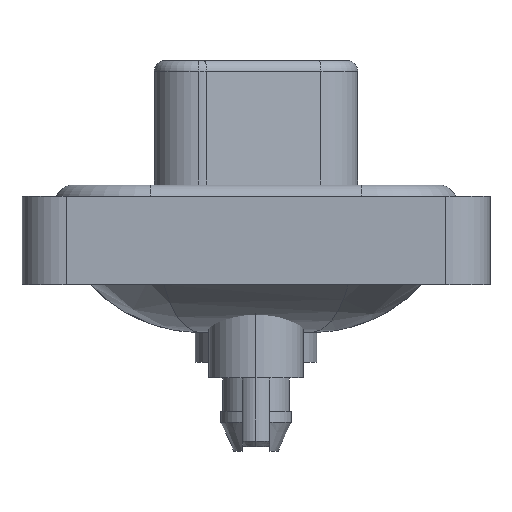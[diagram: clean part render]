
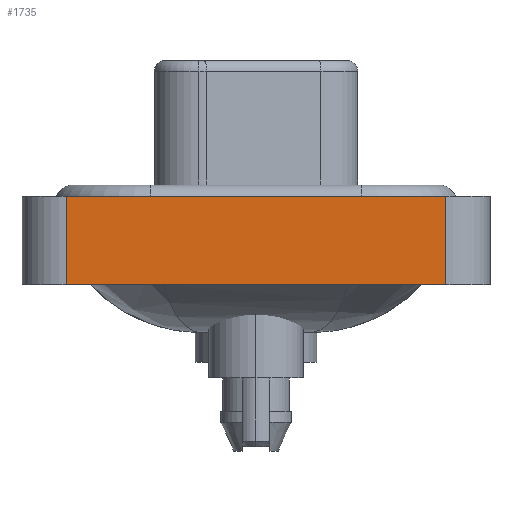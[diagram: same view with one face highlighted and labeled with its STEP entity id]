
A CAD part, left-side view. The second image highlights one B-rep face of the part: STEP entity #1735.
In plain terms, the highlighted planar face has unit normal (-1, 0, 0).
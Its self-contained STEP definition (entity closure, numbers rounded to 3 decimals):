
#616 = EDGE_CURVE ( 'NONE', #1580, #14781, #4866, .T. ) ;
#1580 = VERTEX_POINT ( 'NONE', #3696 ) ;
#1735 = ADVANCED_FACE ( 'NONE', ( #17361 ), #14537, .T. ) ;
#2164 = VERTEX_POINT ( 'NONE', #4454 ) ;
#3252 = DIRECTION ( 'NONE',  ( -1., 0., 0. ) ) ;
#3696 = CARTESIAN_POINT ( 'NONE',  ( -7.25, 8.55, -3.6 ) ) ;
#3746 = CARTESIAN_POINT ( 'NONE',  ( -7.25, -8.55, 0.4 ) ) ;
#3784 = VECTOR ( 'NONE', #11274, 1000. ) ;
#3926 = EDGE_CURVE ( 'NONE', #2164, #17801, #15057, .T. ) ;
#4021 = EDGE_CURVE ( 'NONE', #14781, #17801, #6580, .T. ) ;
#4454 = CARTESIAN_POINT ( 'NONE',  ( -7.25, -8.55, -3.6 ) ) ;
#4730 = CARTESIAN_POINT ( 'NONE',  ( -7.25, 8.55, 0.4 ) ) ;
#4858 = ORIENTED_EDGE ( 'NONE', *, *, #3926, .T. ) ;
#4866 = LINE ( 'NONE', #6640, #7479 ) ;
#5016 = LINE ( 'NONE', #6609, #9259 ) ;
#5276 = ORIENTED_EDGE ( 'NONE', *, *, #616, .F. ) ;
#5667 = ORIENTED_EDGE ( 'NONE', *, *, #4021, .F. ) ;
#6415 = DIRECTION ( 'NONE',  ( 0., -1., 0. ) ) ;
#6580 = LINE ( 'NONE', #3746, #3784 ) ;
#6609 = CARTESIAN_POINT ( 'NONE',  ( -7.25, -8.55, -3.6 ) ) ;
#6640 = CARTESIAN_POINT ( 'NONE',  ( -7.25, 8.55, -3.6 ) ) ;
#7479 = VECTOR ( 'NONE', #18035, 1000. ) ;
#9121 = DIRECTION ( 'NONE',  ( 0., 0., 1. ) ) ;
#9259 = VECTOR ( 'NONE', #6415, 1000. ) ;
#10829 = CARTESIAN_POINT ( 'NONE',  ( -7.25, -8.55, -3.6 ) ) ;
#11274 = DIRECTION ( 'NONE',  ( 0., -1., 0. ) ) ;
#11496 = EDGE_CURVE ( 'NONE', #1580, #2164, #5016, .T. ) ;
#12949 = CARTESIAN_POINT ( 'NONE',  ( -7.25, -8.55, -3.6 ) ) ;
#14537 = PLANE ( 'NONE',  #16606 ) ;
#14781 = VERTEX_POINT ( 'NONE', #4730 ) ;
#14905 = VECTOR ( 'NONE', #9121, 1000. ) ;
#15057 = LINE ( 'NONE', #10829, #14905 ) ;
#15645 = ORIENTED_EDGE ( 'NONE', *, *, #11496, .T. ) ;
#15952 = EDGE_LOOP ( 'NONE', ( #4858, #5667, #5276, #15645 ) ) ;
#16606 = AXIS2_PLACEMENT_3D ( 'NONE', #12949, #3252, #17543 ) ;
#16725 = CARTESIAN_POINT ( 'NONE',  ( -7.25, -8.55, 0.4 ) ) ;
#17361 = FACE_OUTER_BOUND ( 'NONE', #15952, .T. ) ;
#17543 = DIRECTION ( 'NONE',  ( 0., 0., 1. ) ) ;
#17801 = VERTEX_POINT ( 'NONE', #16725 ) ;
#18035 = DIRECTION ( 'NONE',  ( 0., 0., 1. ) ) ;
